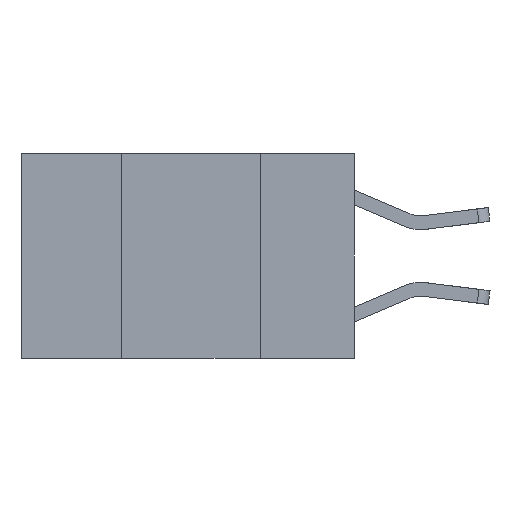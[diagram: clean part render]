
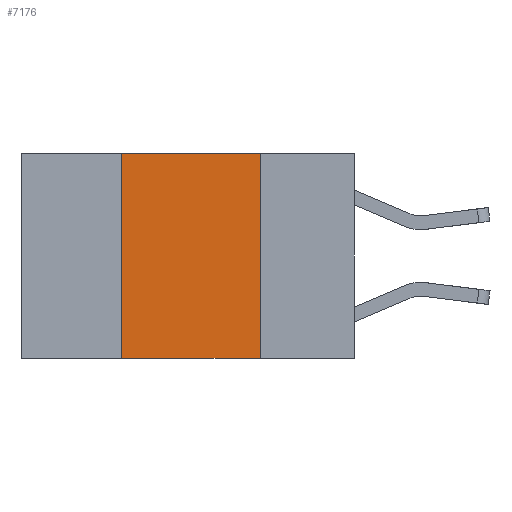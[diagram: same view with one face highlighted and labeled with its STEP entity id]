
A CAD part, left-side view. The second image highlights one B-rep face of the part: STEP entity #7176.
In plain terms, the highlighted planar face has unit normal (-1, 0, 0).
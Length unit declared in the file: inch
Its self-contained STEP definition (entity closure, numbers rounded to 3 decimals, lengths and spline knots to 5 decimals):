
#847 = VECTOR ( 'NONE', #9301, 39.37008 ) ;
#958 = CARTESIAN_POINT ( 'NONE',  ( 0., 0.17, 0. ) ) ;
#1473 = LINE ( 'NONE', #9263, #10170 ) ;
#2490 = DIRECTION ( 'NONE',  ( 0., 0., 1. ) ) ;
#2496 = DIRECTION ( 'NONE',  ( 0., -1., 0. ) ) ;
#3426 = ORIENTED_EDGE ( 'NONE', *, *, #3671, .F. ) ;
#3671 = EDGE_CURVE ( 'NONE', #9624, #3934, #10096, .T. ) ;
#3723 = ORIENTED_EDGE ( 'NONE', *, *, #7423, .F. ) ;
#3934 = VERTEX_POINT ( 'NONE', #958 ) ;
#4466 = VECTOR ( 'NONE', #2490, 39.37008 ) ;
#4804 = DIRECTION ( 'NONE',  ( 0., 0., -1. ) ) ;
#5092 = CARTESIAN_POINT ( 'NONE',  ( 0., 0.6, -0.37 ) ) ;
#5768 = ORIENTED_EDGE ( 'NONE', *, *, #10292, .F. ) ;
#5995 = VECTOR ( 'NONE', #2496, 39.37008 ) ;
#6094 = VERTEX_POINT ( 'NONE', #9049 ) ;
#6136 = CARTESIAN_POINT ( 'NONE',  ( 0., 0.6, 0. ) ) ;
#6924 = CARTESIAN_POINT ( 'NONE',  ( 0., 0.42, 0. ) ) ;
#6987 = CARTESIAN_POINT ( 'NONE',  ( 0., 0.42, 0. ) ) ;
#7176 = ADVANCED_FACE ( 'NONE', ( #8278 ), #7425, .F. ) ;
#7349 = EDGE_CURVE ( 'NONE', #6094, #7685, #9960, .T. ) ;
#7423 = EDGE_CURVE ( 'NONE', #6094, #9624, #11274, .T. ) ;
#7425 = PLANE ( 'NONE',  #10654 ) ;
#7685 = VERTEX_POINT ( 'NONE', #11126 ) ;
#8097 = ORIENTED_EDGE ( 'NONE', *, *, #7349, .T. ) ;
#8221 = CARTESIAN_POINT ( 'NONE',  ( 0., 0.6, 0. ) ) ;
#8278 = FACE_OUTER_BOUND ( 'NONE', #8764, .T. ) ;
#8764 = EDGE_LOOP ( 'NONE', ( #5768, #3426, #3723, #8097 ) ) ;
#9049 = CARTESIAN_POINT ( 'NONE',  ( 0., 0.42, -0.37 ) ) ;
#9263 = CARTESIAN_POINT ( 'NONE',  ( 0., 0.17, 0. ) ) ;
#9301 = DIRECTION ( 'NONE',  ( 0., -1., 0. ) ) ;
#9624 = VERTEX_POINT ( 'NONE', #6924 ) ;
#9803 = DIRECTION ( 'NONE',  ( 1., 0., 0. ) ) ;
#9960 = LINE ( 'NONE', #5092, #847 ) ;
#10021 = DIRECTION ( 'NONE',  ( 0., 0., -1. ) ) ;
#10096 = LINE ( 'NONE', #6136, #5995 ) ;
#10170 = VECTOR ( 'NONE', #10021, 39.37008 ) ;
#10292 = EDGE_CURVE ( 'NONE', #3934, #7685, #1473, .T. ) ;
#10654 = AXIS2_PLACEMENT_3D ( 'NONE', #8221, #9803, #4804 ) ;
#11126 = CARTESIAN_POINT ( 'NONE',  ( 0., 0.17, -0.37 ) ) ;
#11274 = LINE ( 'NONE', #6987, #4466 ) ;
